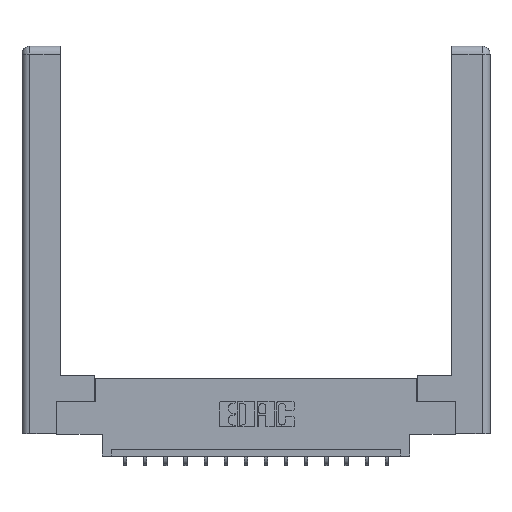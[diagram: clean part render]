
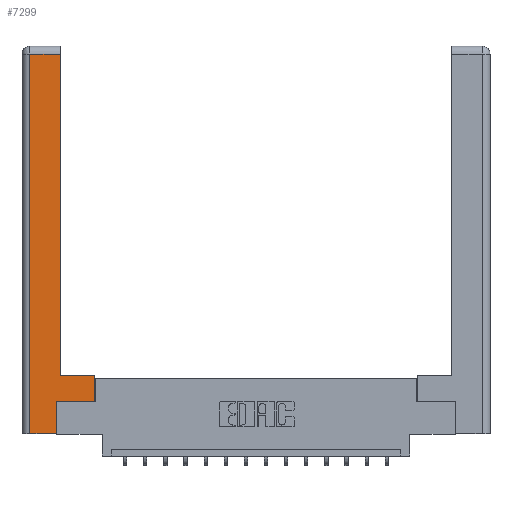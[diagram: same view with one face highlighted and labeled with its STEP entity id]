
A CAD part, top view. The second image highlights one B-rep face of the part: STEP entity #7299.
In plain terms, the highlighted planar face has unit normal (0, 0, 1).
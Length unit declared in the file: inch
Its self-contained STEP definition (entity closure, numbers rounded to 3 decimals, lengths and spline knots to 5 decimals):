
#545 = DIRECTION ( 'NONE',  ( -1., 0., 0. ) ) ;
#656 = LINE ( 'NONE', #11439, #14712 ) ;
#993 = VERTEX_POINT ( 'NONE', #16473 ) ;
#1285 = ORIENTED_EDGE ( 'NONE', *, *, #12151, .T. ) ;
#1325 = LINE ( 'NONE', #6866, #13952 ) ;
#1520 = VECTOR ( 'NONE', #545, 39.37008 ) ;
#2290 = DIRECTION ( 'NONE',  ( 0., 1., 0. ) ) ;
#2364 = PLANE ( 'NONE',  #3676 ) ;
#2384 = DIRECTION ( 'NONE',  ( 0., 1., 0. ) ) ;
#2475 = CARTESIAN_POINT ( 'NONE',  ( 0., 0., 0. ) ) ;
#2627 = DIRECTION ( 'NONE',  ( 0., 1., 0. ) ) ;
#2653 = EDGE_CURVE ( 'NONE', #993, #3666, #7176, .T. ) ;
#3101 = LINE ( 'NONE', #5677, #14128 ) ;
#3115 = VERTEX_POINT ( 'NONE', #4732 ) ;
#3328 = ORIENTED_EDGE ( 'NONE', *, *, #10005, .T. ) ;
#3423 = VECTOR ( 'NONE', #2290, 39.37008 ) ;
#3637 = ORIENTED_EDGE ( 'NONE', *, *, #14256, .T. ) ;
#3666 = VERTEX_POINT ( 'NONE', #15021 ) ;
#3676 = AXIS2_PLACEMENT_3D ( 'NONE', #2475, #12923, #14452 ) ;
#4239 = CARTESIAN_POINT ( 'NONE',  ( 0.565, 0.245, 0. ) ) ;
#4304 = FACE_OUTER_BOUND ( 'NONE', #5697, .T. ) ;
#4413 = DIRECTION ( 'NONE',  ( 1., 0., 0. ) ) ;
#4450 = LINE ( 'NONE', #15244, #3423 ) ;
#4732 = CARTESIAN_POINT ( 'NONE',  ( 0.265, 0., 0. ) ) ;
#5677 = CARTESIAN_POINT ( 'NONE',  ( 0.0615, 0., 0. ) ) ;
#5697 = EDGE_LOOP ( 'NONE', ( #3328, #8393, #11588, #12181, #1285, #15787, #3637, #15844 ) ) ;
#5757 = DIRECTION ( 'NONE',  ( 0., -1., 0. ) ) ;
#6147 = VECTOR ( 'NONE', #15434, 39.37008 ) ;
#6233 = CARTESIAN_POINT ( 'NONE',  ( 0.565, 0.245, 0. ) ) ;
#6276 = LINE ( 'NONE', #4239, #13438 ) ;
#6459 = VERTEX_POINT ( 'NONE', #14744 ) ;
#6866 = CARTESIAN_POINT ( 'NONE',  ( 0.265, 0., 0. ) ) ;
#7020 = VECTOR ( 'NONE', #2627, 39.37008 ) ;
#7176 = LINE ( 'NONE', #14902, #1520 ) ;
#7299 = ADVANCED_FACE ( 'NONE', ( #4304 ), #2364, .F. ) ;
#7404 = CARTESIAN_POINT ( 'NONE',  ( 0.265, 0.245, 0. ) ) ;
#8383 = VERTEX_POINT ( 'NONE', #6233 ) ;
#8393 = ORIENTED_EDGE ( 'NONE', *, *, #11558, .T. ) ;
#9394 = VERTEX_POINT ( 'NONE', #15192 ) ;
#9847 = EDGE_CURVE ( 'NONE', #13266, #3115, #1325, .T. ) ;
#10005 = EDGE_CURVE ( 'NONE', #3666, #9394, #12742, .T. ) ;
#10847 = LINE ( 'NONE', #15320, #6147 ) ;
#11439 = CARTESIAN_POINT ( 'NONE',  ( 0.265, 0.245, 0. ) ) ;
#11462 = EDGE_CURVE ( 'NONE', #6459, #13266, #3101, .T. ) ;
#11558 = EDGE_CURVE ( 'NONE', #9394, #6459, #10847, .T. ) ;
#11588 = ORIENTED_EDGE ( 'NONE', *, *, #11462, .T. ) ;
#12151 = EDGE_CURVE ( 'NONE', #3115, #15416, #656, .T. ) ;
#12181 = ORIENTED_EDGE ( 'NONE', *, *, #9847, .T. ) ;
#12350 = CARTESIAN_POINT ( 'NONE',  ( 0.0615, 0., 0. ) ) ;
#12742 = LINE ( 'NONE', #14257, #7020 ) ;
#12923 = DIRECTION ( 'NONE',  ( 0., 0., -1. ) ) ;
#13266 = VERTEX_POINT ( 'NONE', #12350 ) ;
#13376 = EDGE_CURVE ( 'NONE', #15416, #8383, #6276, .T. ) ;
#13438 = VECTOR ( 'NONE', #4413, 39.37008 ) ;
#13952 = VECTOR ( 'NONE', #16857, 39.37008 ) ;
#14128 = VECTOR ( 'NONE', #5757, 39.37008 ) ;
#14256 = EDGE_CURVE ( 'NONE', #8383, #993, #4450, .T. ) ;
#14257 = CARTESIAN_POINT ( 'NONE',  ( 0.295, 3., 0. ) ) ;
#14452 = DIRECTION ( 'NONE',  ( -1., 0., 0. ) ) ;
#14712 = VECTOR ( 'NONE', #2384, 39.37008 ) ;
#14744 = CARTESIAN_POINT ( 'NONE',  ( 0.0615, 2.94, 0. ) ) ;
#14902 = CARTESIAN_POINT ( 'NONE',  ( 0.295, 0.45, 0. ) ) ;
#15021 = CARTESIAN_POINT ( 'NONE',  ( 0.295, 0.45, 0. ) ) ;
#15192 = CARTESIAN_POINT ( 'NONE',  ( 0.295, 2.94, 0. ) ) ;
#15244 = CARTESIAN_POINT ( 'NONE',  ( 0.565, 0.45, 0. ) ) ;
#15320 = CARTESIAN_POINT ( 'NONE',  ( 0.0615, 2.94, 0. ) ) ;
#15416 = VERTEX_POINT ( 'NONE', #7404 ) ;
#15434 = DIRECTION ( 'NONE',  ( -1., 0., 0. ) ) ;
#15787 = ORIENTED_EDGE ( 'NONE', *, *, #13376, .T. ) ;
#15844 = ORIENTED_EDGE ( 'NONE', *, *, #2653, .T. ) ;
#16473 = CARTESIAN_POINT ( 'NONE',  ( 0.565, 0.45, 0. ) ) ;
#16857 = DIRECTION ( 'NONE',  ( 1., 0., 0. ) ) ;
